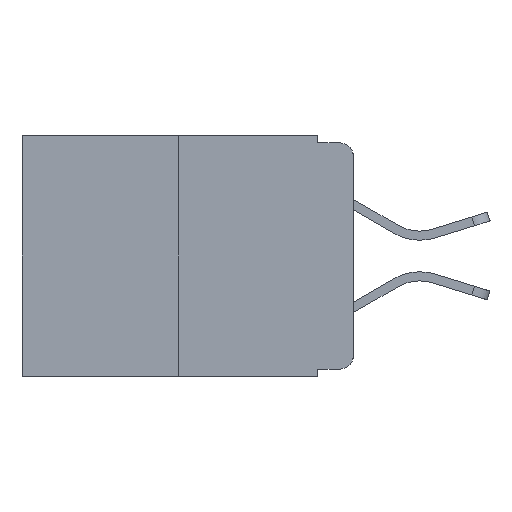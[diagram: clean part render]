
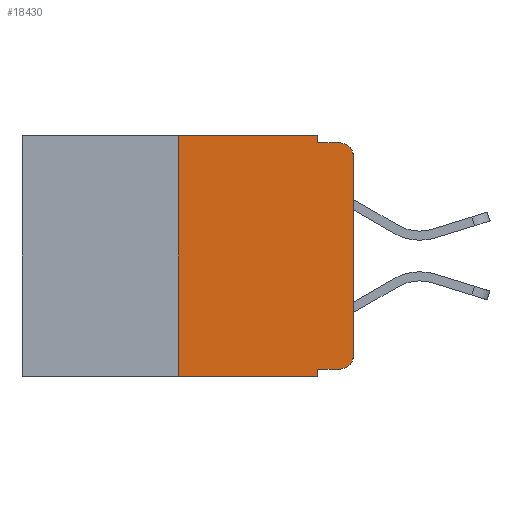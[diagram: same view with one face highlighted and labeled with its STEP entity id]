
A CAD part, left-side view. The second image highlights one B-rep face of the part: STEP entity #18430.
In plain terms, the highlighted planar face has unit normal (-1, 0, 0).
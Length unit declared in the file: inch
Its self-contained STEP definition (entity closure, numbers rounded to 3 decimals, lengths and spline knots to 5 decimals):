
#169 = CIRCLE ( 'NONE', #4094, 0.02 ) ;
#277 = CARTESIAN_POINT ( 'NONE',  ( 0., 0.25, 0. ) ) ;
#532 = ORIENTED_EDGE ( 'NONE', *, *, #17865, .F. ) ;
#740 = DIRECTION ( 'NONE',  ( 0., 0., -1. ) ) ;
#802 = EDGE_CURVE ( 'NONE', #10594, #18239, #2300, .T. ) ;
#837 = DIRECTION ( 'NONE',  ( 0., -1., 0. ) ) ;
#898 = CARTESIAN_POINT ( 'NONE',  ( 0., 0.02, -0.333 ) ) ;
#1005 = DIRECTION ( 'NONE',  ( 0., -1., 0. ) ) ;
#1417 = VERTEX_POINT ( 'NONE', #277 ) ;
#1443 = CARTESIAN_POINT ( 'NONE',  ( 0., 0.051, -0.01 ) ) ;
#2300 = LINE ( 'NONE', #11935, #10440 ) ;
#2384 = CARTESIAN_POINT ( 'NONE',  ( 0., 0.051, 0. ) ) ;
#2591 = CARTESIAN_POINT ( 'NONE',  ( 0., 0., 0. ) ) ;
#2791 = DIRECTION ( 'NONE',  ( 0., 0., -1. ) ) ;
#3144 = LINE ( 'NONE', #17799, #12954 ) ;
#3209 = CARTESIAN_POINT ( 'NONE',  ( 0., 0.051, -0.343 ) ) ;
#3359 = VERTEX_POINT ( 'NONE', #12961 ) ;
#3879 = ORIENTED_EDGE ( 'NONE', *, *, #17883, .T. ) ;
#3949 = ORIENTED_EDGE ( 'NONE', *, *, #16149, .T. ) ;
#4094 = AXIS2_PLACEMENT_3D ( 'NONE', #15985, #14297, #12651 ) ;
#4107 = ORIENTED_EDGE ( 'NONE', *, *, #12815, .F. ) ;
#6070 = LINE ( 'NONE', #6281, #18252 ) ;
#6281 = CARTESIAN_POINT ( 'NONE',  ( 0., 0.051, 0. ) ) ;
#6460 = DIRECTION ( 'NONE',  ( 0., 0., -1. ) ) ;
#6551 = AXIS2_PLACEMENT_3D ( 'NONE', #20069, #15528, #2791 ) ;
#6590 = EDGE_CURVE ( 'NONE', #20208, #16118, #20122, .T. ) ;
#6983 = VECTOR ( 'NONE', #16754, 39.37008 ) ;
#7072 = CIRCLE ( 'NONE', #19044, 0.02 ) ;
#7076 = ORIENTED_EDGE ( 'NONE', *, *, #6590, .T. ) ;
#8350 = LINE ( 'NONE', #10176, #13965 ) ;
#8443 = VECTOR ( 'NONE', #837, 39.37008 ) ;
#8476 = ORIENTED_EDGE ( 'NONE', *, *, #802, .F. ) ;
#9093 = DIRECTION ( 'NONE',  ( 0., 0., -1. ) ) ;
#9147 = CARTESIAN_POINT ( 'NONE',  ( 0., 0.25, -0.343 ) ) ;
#9496 = VERTEX_POINT ( 'NONE', #9917 ) ;
#9917 = CARTESIAN_POINT ( 'NONE',  ( 0., 0.02, -0.01 ) ) ;
#10130 = DIRECTION ( 'NONE',  ( 0., -1., 0. ) ) ;
#10176 = CARTESIAN_POINT ( 'NONE',  ( 0., 0.051, -0.333 ) ) ;
#10440 = VECTOR ( 'NONE', #740, 39.37008 ) ;
#10469 = ORIENTED_EDGE ( 'NONE', *, *, #12542, .T. ) ;
#10514 = DIRECTION ( 'NONE',  ( 0., 0., 1. ) ) ;
#10594 = VERTEX_POINT ( 'NONE', #2384 ) ;
#11078 = VERTEX_POINT ( 'NONE', #898 ) ;
#11140 = LINE ( 'NONE', #11992, #6983 ) ;
#11935 = CARTESIAN_POINT ( 'NONE',  ( 0., 0.051, 0. ) ) ;
#11992 = CARTESIAN_POINT ( 'NONE',  ( 0., 0.25, 0. ) ) ;
#12524 = CARTESIAN_POINT ( 'NONE',  ( 0., 0.02, -0.03 ) ) ;
#12542 = EDGE_CURVE ( 'NONE', #3359, #11078, #8350, .T. ) ;
#12651 = DIRECTION ( 'NONE',  ( 0., 0., -1. ) ) ;
#12782 = ORIENTED_EDGE ( 'NONE', *, *, #14860, .T. ) ;
#12815 = EDGE_CURVE ( 'NONE', #1417, #10594, #3144, .T. ) ;
#12889 = FACE_OUTER_BOUND ( 'NONE', #16656, .T. ) ;
#12954 = VECTOR ( 'NONE', #10130, 39.37008 ) ;
#12961 = CARTESIAN_POINT ( 'NONE',  ( 0., 0.051, -0.333 ) ) ;
#13253 = CARTESIAN_POINT ( 'NONE',  ( 0., 0.473, -0.343 ) ) ;
#13692 = CARTESIAN_POINT ( 'NONE',  ( 0., 0., -0.313 ) ) ;
#13728 = ORIENTED_EDGE ( 'NONE', *, *, #16430, .F. ) ;
#13965 = VECTOR ( 'NONE', #1005, 39.37008 ) ;
#14248 = CARTESIAN_POINT ( 'NONE',  ( 0., 0., -0.03 ) ) ;
#14262 = VERTEX_POINT ( 'NONE', #14248 ) ;
#14297 = DIRECTION ( 'NONE',  ( -1., 0., 0. ) ) ;
#14585 = VERTEX_POINT ( 'NONE', #13692 ) ;
#14860 = EDGE_CURVE ( 'NONE', #11078, #14585, #169, .T. ) ;
#15268 = VECTOR ( 'NONE', #10514, 39.37008 ) ;
#15528 = DIRECTION ( 'NONE',  ( 1., 0., 0. ) ) ;
#15985 = CARTESIAN_POINT ( 'NONE',  ( 0., 0.02, -0.313 ) ) ;
#16038 = LINE ( 'NONE', #1443, #19188 ) ;
#16118 = VERTEX_POINT ( 'NONE', #3209 ) ;
#16149 = EDGE_CURVE ( 'NONE', #14262, #9496, #7072, .T. ) ;
#16430 = EDGE_CURVE ( 'NONE', #3359, #16118, #6070, .T. ) ;
#16656 = EDGE_LOOP ( 'NONE', ( #3879, #3949, #18524, #8476, #4107, #532, #7076, #13728, #10469, #12782 ) ) ;
#16754 = DIRECTION ( 'NONE',  ( 0., 0., 1. ) ) ;
#17225 = DIRECTION ( 'NONE',  ( -1., 0., 0. ) ) ;
#17440 = EDGE_CURVE ( 'NONE', #18239, #9496, #16038, .T. ) ;
#17767 = CARTESIAN_POINT ( 'NONE',  ( 0., 0.051, -0.01 ) ) ;
#17799 = CARTESIAN_POINT ( 'NONE',  ( 0., 0.473, 0. ) ) ;
#17865 = EDGE_CURVE ( 'NONE', #20208, #1417, #11140, .T. ) ;
#17883 = EDGE_CURVE ( 'NONE', #14585, #14262, #19412, .T. ) ;
#18239 = VERTEX_POINT ( 'NONE', #17767 ) ;
#18252 = VECTOR ( 'NONE', #9093, 39.37008 ) ;
#18394 = DIRECTION ( 'NONE',  ( 0., -1., 0. ) ) ;
#18430 = ADVANCED_FACE ( 'NONE', ( #12889 ), #19619, .F. ) ;
#18524 = ORIENTED_EDGE ( 'NONE', *, *, #17440, .F. ) ;
#19044 = AXIS2_PLACEMENT_3D ( 'NONE', #12524, #17225, #6460 ) ;
#19188 = VECTOR ( 'NONE', #18394, 39.37008 ) ;
#19412 = LINE ( 'NONE', #2591, #15268 ) ;
#19619 = PLANE ( 'NONE',  #6551 ) ;
#20069 = CARTESIAN_POINT ( 'NONE',  ( 0., 0.473, 0. ) ) ;
#20122 = LINE ( 'NONE', #13253, #8443 ) ;
#20208 = VERTEX_POINT ( 'NONE', #9147 ) ;
